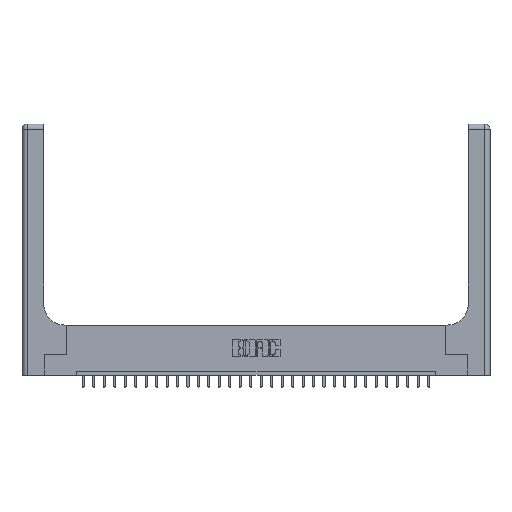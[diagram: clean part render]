
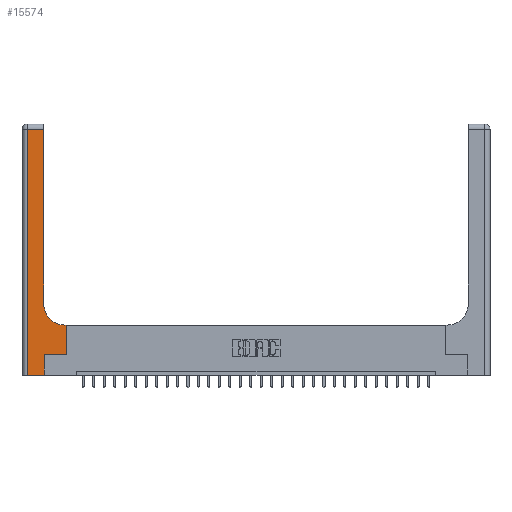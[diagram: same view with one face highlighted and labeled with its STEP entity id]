
A CAD part, top view. The second image highlights one B-rep face of the part: STEP entity #15574.
In plain terms, the highlighted planar face has unit normal (0, 0, 1).
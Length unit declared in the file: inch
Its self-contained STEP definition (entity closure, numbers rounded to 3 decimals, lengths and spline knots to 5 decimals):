
#616 = VERTEX_POINT ( 'NONE', #12381 ) ;
#620 = DIRECTION ( 'NONE',  ( 0., -1., 0. ) ) ;
#726 = LINE ( 'NONE', #2767, #8040 ) ;
#1161 = DIRECTION ( 'NONE',  ( 1., 0., 0. ) ) ;
#2523 = CARTESIAN_POINT ( 'NONE',  ( 0.528, 0.25, 0.37 ) ) ;
#2767 = CARTESIAN_POINT ( 'NONE',  ( 0.26, 3., 0.37 ) ) ;
#3217 = CARTESIAN_POINT ( 'NONE',  ( 0., 0., 0.37 ) ) ;
#3498 = VERTEX_POINT ( 'NONE', #4672 ) ;
#3809 = VECTOR ( 'NONE', #1161, 39.37008 ) ;
#3859 = LINE ( 'NONE', #17589, #17471 ) ;
#4672 = CARTESIAN_POINT ( 'NONE',  ( 0.528, 0.6, 0.37 ) ) ;
#6135 = DIRECTION ( 'NONE',  ( 0., 0., -1. ) ) ;
#6773 = DIRECTION ( 'NONE',  ( 0., 1., 0. ) ) ;
#6944 = EDGE_CURVE ( 'NONE', #9059, #23248, #12891, .T. ) ;
#6974 = VECTOR ( 'NONE', #19763, 39.37008 ) ;
#7085 = ORIENTED_EDGE ( 'NONE', *, *, #22362, .T. ) ;
#7322 = LINE ( 'NONE', #2523, #6974 ) ;
#7363 = CIRCLE ( 'NONE', #14407, 0.25 ) ;
#7704 = EDGE_CURVE ( 'NONE', #3498, #616, #3859, .T. ) ;
#8040 = VECTOR ( 'NONE', #6773, 39.37008 ) ;
#8100 = ORIENTED_EDGE ( 'NONE', *, *, #6944, .T. ) ;
#8487 = LINE ( 'NONE', #9961, #3809 ) ;
#8654 = CARTESIAN_POINT ( 'NONE',  ( 0.06, 0., 0.37 ) ) ;
#9059 = VERTEX_POINT ( 'NONE', #8654 ) ;
#9385 = ORIENTED_EDGE ( 'NONE', *, *, #24092, .T. ) ;
#9570 = VECTOR ( 'NONE', #26527, 39.37008 ) ;
#9820 = DIRECTION ( 'NONE',  ( -1., 0., 0. ) ) ;
#9949 = VECTOR ( 'NONE', #9820, 39.37008 ) ;
#9961 = CARTESIAN_POINT ( 'NONE',  ( 0.265, 0.25, 0.37 ) ) ;
#10191 = VECTOR ( 'NONE', #620, 39.37008 ) ;
#10320 = EDGE_CURVE ( 'NONE', #26686, #23664, #726, .T. ) ;
#11318 = VERTEX_POINT ( 'NONE', #12685 ) ;
#11543 = LINE ( 'NONE', #27397, #24424 ) ;
#11683 = CARTESIAN_POINT ( 'NONE',  ( 0.26, 2.94, 0.37 ) ) ;
#12381 = CARTESIAN_POINT ( 'NONE',  ( 0.51, 0.6, 0.37 ) ) ;
#12468 = ORIENTED_EDGE ( 'NONE', *, *, #7704, .T. ) ;
#12685 = CARTESIAN_POINT ( 'NONE',  ( 0.06, 2.94, 0.37 ) ) ;
#12739 = ORIENTED_EDGE ( 'NONE', *, *, #10320, .T. ) ;
#12891 = LINE ( 'NONE', #3217, #9570 ) ;
#13014 = DIRECTION ( 'NONE',  ( 0., 0., -1. ) ) ;
#14407 = AXIS2_PLACEMENT_3D ( 'NONE', #19286, #13014, #21315 ) ;
#14828 = CARTESIAN_POINT ( 'NONE',  ( 0., 3., 0.37 ) ) ;
#15221 = EDGE_CURVE ( 'NONE', #15420, #3498, #7322, .T. ) ;
#15420 = VERTEX_POINT ( 'NONE', #24826 ) ;
#15574 = ADVANCED_FACE ( 'NONE', ( #24184 ), #25191, .F. ) ;
#16528 = ORIENTED_EDGE ( 'NONE', *, *, #17010, .T. ) ;
#16974 = CARTESIAN_POINT ( 'NONE',  ( 0.265, 0.25, 0.37 ) ) ;
#17010 = EDGE_CURVE ( 'NONE', #23248, #21917, #11543, .T. ) ;
#17374 = CARTESIAN_POINT ( 'NONE',  ( 0.26, 0.85, 0.37 ) ) ;
#17471 = VECTOR ( 'NONE', #19709, 39.37008 ) ;
#17589 = CARTESIAN_POINT ( 'NONE',  ( 0.26, 0.6, 0.37 ) ) ;
#18338 = CARTESIAN_POINT ( 'NONE',  ( 0., 2.94, 0.37 ) ) ;
#18911 = DIRECTION ( 'NONE',  ( -1., 0., 0. ) ) ;
#19093 = CARTESIAN_POINT ( 'NONE',  ( 0.265, 0., 0.37 ) ) ;
#19286 = CARTESIAN_POINT ( 'NONE',  ( 0.51, 0.85, 0.37 ) ) ;
#19709 = DIRECTION ( 'NONE',  ( -1., 0., 0. ) ) ;
#19763 = DIRECTION ( 'NONE',  ( 0., 1., 0. ) ) ;
#20040 = ORIENTED_EDGE ( 'NONE', *, *, #27189, .T. ) ;
#21315 = DIRECTION ( 'NONE',  ( 1., 0., 0. ) ) ;
#21765 = ORIENTED_EDGE ( 'NONE', *, *, #24404, .T. ) ;
#21917 = VERTEX_POINT ( 'NONE', #16974 ) ;
#22362 = EDGE_CURVE ( 'NONE', #23664, #11318, #26812, .T. ) ;
#22731 = EDGE_LOOP ( 'NONE', ( #12739, #7085, #9385, #8100, #16528, #21765, #25561, #12468, #20040 ) ) ;
#22773 = LINE ( 'NONE', #23589, #10191 ) ;
#23248 = VERTEX_POINT ( 'NONE', #19093 ) ;
#23589 = CARTESIAN_POINT ( 'NONE',  ( 0.06, 3., 0.37 ) ) ;
#23664 = VERTEX_POINT ( 'NONE', #11683 ) ;
#24092 = EDGE_CURVE ( 'NONE', #11318, #9059, #22773, .T. ) ;
#24184 = FACE_OUTER_BOUND ( 'NONE', #22731, .T. ) ;
#24404 = EDGE_CURVE ( 'NONE', #21917, #15420, #8487, .T. ) ;
#24424 = VECTOR ( 'NONE', #25282, 39.37008 ) ;
#24826 = CARTESIAN_POINT ( 'NONE',  ( 0.528, 0.25, 0.37 ) ) ;
#25191 = PLANE ( 'NONE',  #25311 ) ;
#25282 = DIRECTION ( 'NONE',  ( 0., 1., 0. ) ) ;
#25311 = AXIS2_PLACEMENT_3D ( 'NONE', #14828, #6135, #18911 ) ;
#25561 = ORIENTED_EDGE ( 'NONE', *, *, #15221, .T. ) ;
#26527 = DIRECTION ( 'NONE',  ( 1., 0., 0. ) ) ;
#26686 = VERTEX_POINT ( 'NONE', #17374 ) ;
#26812 = LINE ( 'NONE', #18338, #9949 ) ;
#27189 = EDGE_CURVE ( 'NONE', #616, #26686, #7363, .T. ) ;
#27397 = CARTESIAN_POINT ( 'NONE',  ( 0.265, 0., 0.37 ) ) ;
